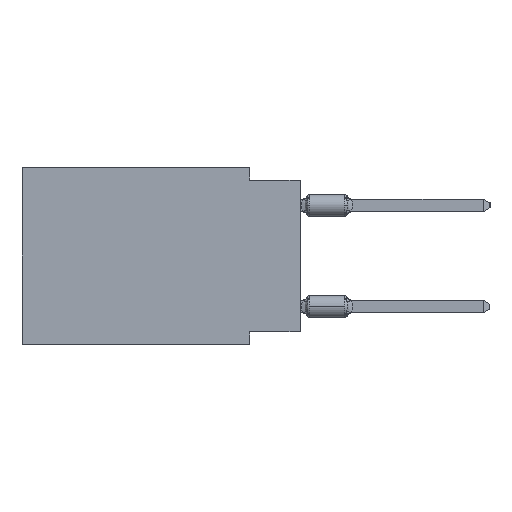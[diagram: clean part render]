
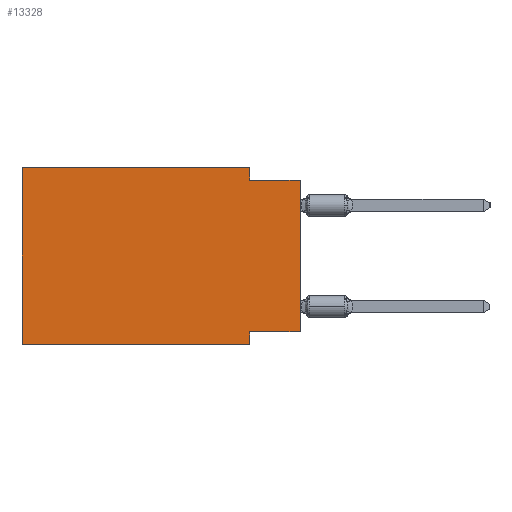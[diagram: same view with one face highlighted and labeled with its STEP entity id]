
A CAD part, left-side view. The second image highlights one B-rep face of the part: STEP entity #13328.
In plain terms, the highlighted planar face has unit normal (-1, 0, 0).
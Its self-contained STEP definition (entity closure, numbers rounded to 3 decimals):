
#171 = EDGE_CURVE ( 'NONE', #12827, #14837, #16264, .T. ) ;
#494 = ORIENTED_EDGE ( 'NONE', *, *, #13392, .T. ) ;
#598 = CARTESIAN_POINT ( 'NONE',  ( 0., 2.54, -8.89 ) ) ;
#1529 = CARTESIAN_POINT ( 'NONE',  ( 0., 2.54, 0. ) ) ;
#1621 = VECTOR ( 'NONE', #5494, 1000. ) ;
#1900 = VECTOR ( 'NONE', #22730, 1000. ) ;
#3927 = DIRECTION ( 'NONE',  ( 0., -1., 0. ) ) ;
#4843 = VECTOR ( 'NONE', #5714, 1000. ) ;
#5494 = DIRECTION ( 'NONE',  ( 0., 1., 0. ) ) ;
#5714 = DIRECTION ( 'NONE',  ( 0., 0., 1. ) ) ;
#6247 = EDGE_CURVE ( 'NONE', #13101, #26703, #17950, .T. ) ;
#6774 = ORIENTED_EDGE ( 'NONE', *, *, #16978, .F. ) ;
#7565 = CARTESIAN_POINT ( 'NONE',  ( 0., 13.97, 0. ) ) ;
#9216 = DIRECTION ( 'NONE',  ( 0., 0., 1. ) ) ;
#10276 = FACE_OUTER_BOUND ( 'NONE', #20523, .T. ) ;
#10354 = ORIENTED_EDGE ( 'NONE', *, *, #6247, .F. ) ;
#10877 = CARTESIAN_POINT ( 'NONE',  ( 0., 13.97, 0. ) ) ;
#11396 = CARTESIAN_POINT ( 'NONE',  ( 0., 13.97, 0. ) ) ;
#11794 = CARTESIAN_POINT ( 'NONE',  ( 0., 0., 0. ) ) ;
#12315 = VECTOR ( 'NONE', #9216, 1000. ) ;
#12827 = VERTEX_POINT ( 'NONE', #7565 ) ;
#13101 = VERTEX_POINT ( 'NONE', #25855 ) ;
#13175 = LINE ( 'NONE', #29883, #22097 ) ;
#13266 = VECTOR ( 'NONE', #3927, 1000. ) ;
#13328 = ADVANCED_FACE ( 'NONE', ( #10276 ), #25019, .F. ) ;
#13392 = EDGE_CURVE ( 'NONE', #31474, #30410, #13175, .T. ) ;
#14238 = LINE ( 'NONE', #11794, #12315 ) ;
#14837 = VERTEX_POINT ( 'NONE', #1529 ) ;
#15229 = ORIENTED_EDGE ( 'NONE', *, *, #171, .F. ) ;
#15624 = DIRECTION ( 'NONE',  ( 1., 0., 0. ) ) ;
#15688 = CARTESIAN_POINT ( 'NONE',  ( 0., 0., -8.255 ) ) ;
#16050 = CARTESIAN_POINT ( 'NONE',  ( 0., 2.54, -0.635 ) ) ;
#16147 = VERTEX_POINT ( 'NONE', #18243 ) ;
#16264 = LINE ( 'NONE', #11396, #24093 ) ;
#16978 = EDGE_CURVE ( 'NONE', #31474, #12827, #27578, .T. ) ;
#17950 = LINE ( 'NONE', #15688, #1621 ) ;
#18163 = EDGE_CURVE ( 'NONE', #14837, #18729, #30027, .T. ) ;
#18195 = CARTESIAN_POINT ( 'NONE',  ( 0., 13.97, 0. ) ) ;
#18243 = CARTESIAN_POINT ( 'NONE',  ( 0., 0., -0.635 ) ) ;
#18383 = EDGE_CURVE ( 'NONE', #18729, #16147, #30815, .T. ) ;
#18729 = VERTEX_POINT ( 'NONE', #16050 ) ;
#20214 = EDGE_CURVE ( 'NONE', #13101, #16147, #14238, .T. ) ;
#20373 = ORIENTED_EDGE ( 'NONE', *, *, #26412, .F. ) ;
#20523 = EDGE_LOOP ( 'NONE', ( #31842, #27626, #27802, #15229, #6774, #494, #20373, #10354 ) ) ;
#21132 = DIRECTION ( 'NONE',  ( 0., -1., 0. ) ) ;
#22097 = VECTOR ( 'NONE', #27920, 1000. ) ;
#22730 = DIRECTION ( 'NONE',  ( 0., 0., -1. ) ) ;
#23245 = CARTESIAN_POINT ( 'NONE',  ( 0., 2.54, -8.89 ) ) ;
#24093 = VECTOR ( 'NONE', #21132, 1000. ) ;
#25019 = PLANE ( 'NONE',  #27785 ) ;
#25182 = DIRECTION ( 'NONE',  ( 0., 0., -1. ) ) ;
#25371 = DIRECTION ( 'NONE',  ( 0., 0., -1. ) ) ;
#25469 = VECTOR ( 'NONE', #25371, 1000. ) ;
#25855 = CARTESIAN_POINT ( 'NONE',  ( 0., 0., -8.255 ) ) ;
#26125 = CARTESIAN_POINT ( 'NONE',  ( 0., 0., -0.635 ) ) ;
#26412 = EDGE_CURVE ( 'NONE', #26703, #30410, #30079, .T. ) ;
#26703 = VERTEX_POINT ( 'NONE', #30809 ) ;
#27069 = CARTESIAN_POINT ( 'NONE',  ( 0., 13.97, -8.89 ) ) ;
#27578 = LINE ( 'NONE', #10877, #4843 ) ;
#27585 = CARTESIAN_POINT ( 'NONE',  ( 0., 2.54, 0. ) ) ;
#27626 = ORIENTED_EDGE ( 'NONE', *, *, #18383, .F. ) ;
#27785 = AXIS2_PLACEMENT_3D ( 'NONE', #18195, #15624, #25182 ) ;
#27802 = ORIENTED_EDGE ( 'NONE', *, *, #18163, .F. ) ;
#27920 = DIRECTION ( 'NONE',  ( 0., -1., 0. ) ) ;
#29883 = CARTESIAN_POINT ( 'NONE',  ( 0., 13.97, -8.89 ) ) ;
#30027 = LINE ( 'NONE', #27585, #1900 ) ;
#30079 = LINE ( 'NONE', #598, #25469 ) ;
#30410 = VERTEX_POINT ( 'NONE', #23245 ) ;
#30809 = CARTESIAN_POINT ( 'NONE',  ( 0., 2.54, -8.255 ) ) ;
#30815 = LINE ( 'NONE', #26125, #13266 ) ;
#31474 = VERTEX_POINT ( 'NONE', #27069 ) ;
#31842 = ORIENTED_EDGE ( 'NONE', *, *, #20214, .T. ) ;
